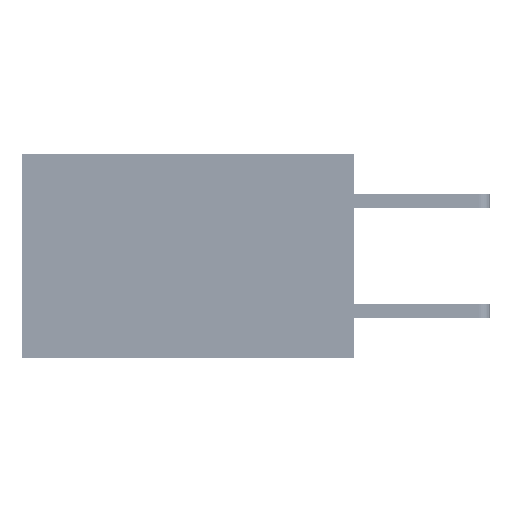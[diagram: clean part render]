
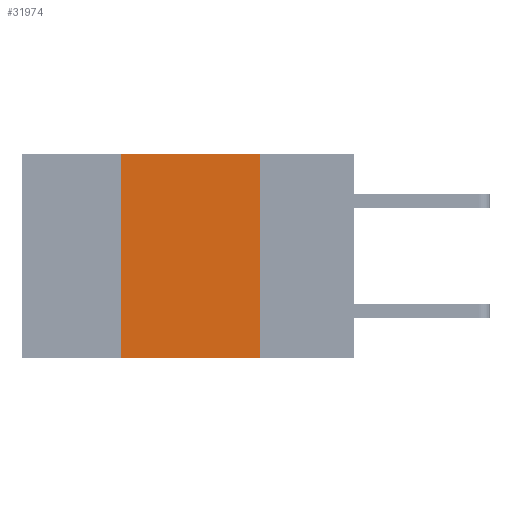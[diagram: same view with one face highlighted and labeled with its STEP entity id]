
A CAD part, left-side view. The second image highlights one B-rep face of the part: STEP entity #31974.
In plain terms, the highlighted planar face has unit normal (-1, 0, 0).
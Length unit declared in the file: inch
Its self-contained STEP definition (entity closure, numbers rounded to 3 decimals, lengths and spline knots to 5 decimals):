
#382 = EDGE_CURVE ( 'NONE', #12324, #12189, #27092, .T. ) ;
#1239 = CARTESIAN_POINT ( 'NONE',  ( 0., 0.42, 0. ) ) ;
#1662 = VERTEX_POINT ( 'NONE', #25303 ) ;
#2133 = CARTESIAN_POINT ( 'NONE',  ( 0., 0.42, 0. ) ) ;
#2710 = CARTESIAN_POINT ( 'NONE',  ( 0., 0.17, 0. ) ) ;
#3350 = CARTESIAN_POINT ( 'NONE',  ( 0., 0.6, 0. ) ) ;
#5285 = ORIENTED_EDGE ( 'NONE', *, *, #9587, .F. ) ;
#7142 = LINE ( 'NONE', #13439, #13433 ) ;
#9587 = EDGE_CURVE ( 'NONE', #14074, #12324, #7142, .T. ) ;
#11229 = EDGE_CURVE ( 'NONE', #1662, #12189, #30027, .T. ) ;
#11896 = VECTOR ( 'NONE', #27080, 39.37008 ) ;
#12189 = VERTEX_POINT ( 'NONE', #17289 ) ;
#12286 = DIRECTION ( 'NONE',  ( 0., -1., 0. ) ) ;
#12324 = VERTEX_POINT ( 'NONE', #32071 ) ;
#13433 = VECTOR ( 'NONE', #12286, 39.37008 ) ;
#13439 = CARTESIAN_POINT ( 'NONE',  ( 0., 0.6, 0. ) ) ;
#13637 = ORIENTED_EDGE ( 'NONE', *, *, #34139, .F. ) ;
#14074 = VERTEX_POINT ( 'NONE', #1239 ) ;
#15300 = VECTOR ( 'NONE', #21718, 39.37008 ) ;
#16829 = PLANE ( 'NONE',  #19845 ) ;
#17289 = CARTESIAN_POINT ( 'NONE',  ( 0., 0.17, -0.37 ) ) ;
#18680 = DIRECTION ( 'NONE',  ( 0., -1., 0. ) ) ;
#19845 = AXIS2_PLACEMENT_3D ( 'NONE', #3350, #40254, #20320 ) ;
#20320 = DIRECTION ( 'NONE',  ( 0., 0., -1. ) ) ;
#20356 = FACE_OUTER_BOUND ( 'NONE', #41002, .T. ) ;
#21718 = DIRECTION ( 'NONE',  ( 0., 0., 1. ) ) ;
#25303 = CARTESIAN_POINT ( 'NONE',  ( 0., 0.42, -0.37 ) ) ;
#25699 = CARTESIAN_POINT ( 'NONE',  ( 0., 0.6, -0.37 ) ) ;
#27080 = DIRECTION ( 'NONE',  ( 0., 0., -1. ) ) ;
#27092 = LINE ( 'NONE', #2710, #11896 ) ;
#27612 = ORIENTED_EDGE ( 'NONE', *, *, #382, .F. ) ;
#28962 = VECTOR ( 'NONE', #18680, 39.37008 ) ;
#30027 = LINE ( 'NONE', #25699, #28962 ) ;
#31974 = ADVANCED_FACE ( 'NONE', ( #20356 ), #16829, .F. ) ;
#32071 = CARTESIAN_POINT ( 'NONE',  ( 0., 0.17, 0. ) ) ;
#34139 = EDGE_CURVE ( 'NONE', #1662, #14074, #39937, .T. ) ;
#36382 = ORIENTED_EDGE ( 'NONE', *, *, #11229, .T. ) ;
#39937 = LINE ( 'NONE', #2133, #15300 ) ;
#40254 = DIRECTION ( 'NONE',  ( 1., 0., 0. ) ) ;
#41002 = EDGE_LOOP ( 'NONE', ( #27612, #5285, #13637, #36382 ) ) ;
